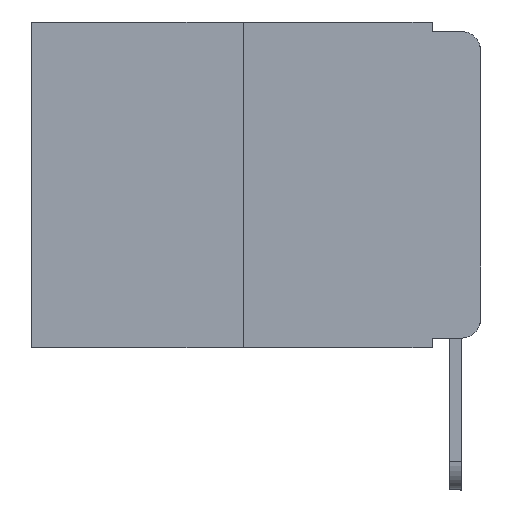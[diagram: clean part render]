
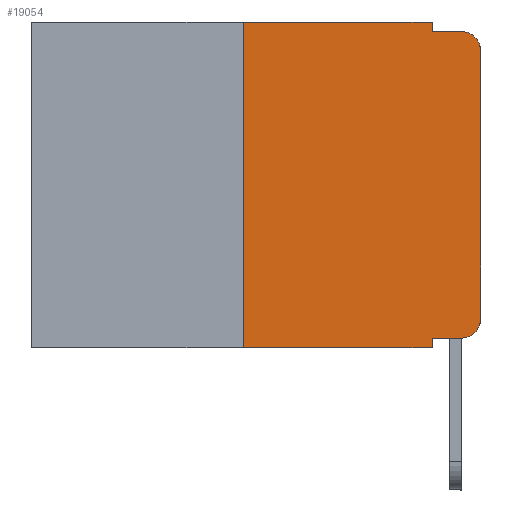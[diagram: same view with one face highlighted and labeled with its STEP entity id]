
A CAD part, left-side view. The second image highlights one B-rep face of the part: STEP entity #19054.
In plain terms, the highlighted planar face has unit normal (-1, 0, 0).
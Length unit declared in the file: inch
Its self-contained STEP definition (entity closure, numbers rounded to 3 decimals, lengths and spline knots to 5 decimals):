
#130 = VECTOR ( 'NONE', #16794, 39.37008 ) ;
#879 = LINE ( 'NONE', #5907, #19585 ) ;
#1122 = VECTOR ( 'NONE', #14082, 39.37008 ) ;
#1178 = VERTEX_POINT ( 'NONE', #13320 ) ;
#1684 = VECTOR ( 'NONE', #13153, 39.37008 ) ;
#2088 = CARTESIAN_POINT ( 'NONE',  ( 0., 0.051, -0.343 ) ) ;
#2218 = DIRECTION ( 'NONE',  ( 0., -1., 0. ) ) ;
#2637 = DIRECTION ( 'NONE',  ( 0., 0., -1. ) ) ;
#2649 = ORIENTED_EDGE ( 'NONE', *, *, #18471, .F. ) ;
#2933 = AXIS2_PLACEMENT_3D ( 'NONE', #17902, #2982, #14634 ) ;
#2982 = DIRECTION ( 'NONE',  ( -1., 0., 0. ) ) ;
#2997 = DIRECTION ( 'NONE',  ( 0., 0., -1. ) ) ;
#3019 = CARTESIAN_POINT ( 'NONE',  ( 0., 0.02, -0.333 ) ) ;
#3171 = VERTEX_POINT ( 'NONE', #12402 ) ;
#3204 = LINE ( 'NONE', #9836, #130 ) ;
#3533 = VECTOR ( 'NONE', #2997, 39.37008 ) ;
#4018 = EDGE_CURVE ( 'NONE', #15065, #11199, #5393, .T. ) ;
#4081 = CARTESIAN_POINT ( 'NONE',  ( 0., 0.051, -0.333 ) ) ;
#4201 = LINE ( 'NONE', #12363, #8523 ) ;
#4437 = VECTOR ( 'NONE', #2218, 39.37008 ) ;
#4520 = CARTESIAN_POINT ( 'NONE',  ( 0., 0.051, 0. ) ) ;
#4882 = VERTEX_POINT ( 'NONE', #17727 ) ;
#5393 = LINE ( 'NONE', #19218, #4437 ) ;
#5612 = DIRECTION ( 'NONE',  ( 0., 0., 1. ) ) ;
#5907 = CARTESIAN_POINT ( 'NONE',  ( 0., 0.051, 0. ) ) ;
#6014 = LINE ( 'NONE', #7534, #1122 ) ;
#6419 = DIRECTION ( 'NONE',  ( 1., 0., 0. ) ) ;
#6488 = CARTESIAN_POINT ( 'NONE',  ( 0., 0.051, -0.01 ) ) ;
#6549 = CARTESIAN_POINT ( 'NONE',  ( 0., 0.02, -0.03 ) ) ;
#6575 = CARTESIAN_POINT ( 'NONE',  ( 0., 0.051, 0. ) ) ;
#6661 = EDGE_CURVE ( 'NONE', #12435, #9947, #6906, .T. ) ;
#6898 = ORIENTED_EDGE ( 'NONE', *, *, #6661, .F. ) ;
#6906 = LINE ( 'NONE', #6488, #1684 ) ;
#7318 = CARTESIAN_POINT ( 'NONE',  ( 0., 0.02, -0.01 ) ) ;
#7534 = CARTESIAN_POINT ( 'NONE',  ( 0., 0.25, 0. ) ) ;
#7578 = CARTESIAN_POINT ( 'NONE',  ( 0., 0.25, -0.343 ) ) ;
#7665 = CARTESIAN_POINT ( 'NONE',  ( 0., 0.25, 0. ) ) ;
#7877 = VERTEX_POINT ( 'NONE', #3019 ) ;
#8114 = ORIENTED_EDGE ( 'NONE', *, *, #13920, .F. ) ;
#8523 = VECTOR ( 'NONE', #5612, 39.37008 ) ;
#9652 = VERTEX_POINT ( 'NONE', #7665 ) ;
#9836 = CARTESIAN_POINT ( 'NONE',  ( 0., 0.473, 0. ) ) ;
#9839 = ORIENTED_EDGE ( 'NONE', *, *, #15367, .T. ) ;
#9947 = VERTEX_POINT ( 'NONE', #7318 ) ;
#10528 = ORIENTED_EDGE ( 'NONE', *, *, #4018, .T. ) ;
#11019 = VECTOR ( 'NONE', #19105, 39.37008 ) ;
#11199 = VERTEX_POINT ( 'NONE', #2088 ) ;
#12363 = CARTESIAN_POINT ( 'NONE',  ( 0., 0., 0. ) ) ;
#12402 = CARTESIAN_POINT ( 'NONE',  ( 0., 0., -0.313 ) ) ;
#12435 = VERTEX_POINT ( 'NONE', #17462 ) ;
#12578 = LINE ( 'NONE', #4081, #11019 ) ;
#12999 = DIRECTION ( 'NONE',  ( 0., 0., -1. ) ) ;
#13153 = DIRECTION ( 'NONE',  ( 0., -1., 0. ) ) ;
#13306 = EDGE_LOOP ( 'NONE', ( #21253, #15072, #6898, #19586, #8114, #2649, #10528, #14712, #9839, #20119 ) ) ;
#13320 = CARTESIAN_POINT ( 'NONE',  ( 0., 0., -0.03 ) ) ;
#13336 = AXIS2_PLACEMENT_3D ( 'NONE', #6549, #14953, #12999 ) ;
#13729 = EDGE_CURVE ( 'NONE', #7877, #3171, #19641, .T. ) ;
#13920 = EDGE_CURVE ( 'NONE', #9652, #18074, #3204, .T. ) ;
#14082 = DIRECTION ( 'NONE',  ( 0., 0., 1. ) ) ;
#14634 = DIRECTION ( 'NONE',  ( 0., 0., -1. ) ) ;
#14712 = ORIENTED_EDGE ( 'NONE', *, *, #18508, .F. ) ;
#14953 = DIRECTION ( 'NONE',  ( -1., 0., 0. ) ) ;
#15065 = VERTEX_POINT ( 'NONE', #7578 ) ;
#15072 = ORIENTED_EDGE ( 'NONE', *, *, #18579, .T. ) ;
#15367 = EDGE_CURVE ( 'NONE', #4882, #7877, #12578, .T. ) ;
#16794 = DIRECTION ( 'NONE',  ( 0., -1., 0. ) ) ;
#16840 = EDGE_CURVE ( 'NONE', #18074, #12435, #18342, .T. ) ;
#17462 = CARTESIAN_POINT ( 'NONE',  ( 0., 0.051, -0.01 ) ) ;
#17727 = CARTESIAN_POINT ( 'NONE',  ( 0., 0.051, -0.333 ) ) ;
#17863 = DIRECTION ( 'NONE',  ( 0., 0., -1. ) ) ;
#17902 = CARTESIAN_POINT ( 'NONE',  ( 0., 0.02, -0.313 ) ) ;
#18074 = VERTEX_POINT ( 'NONE', #4520 ) ;
#18342 = LINE ( 'NONE', #6575, #3533 ) ;
#18471 = EDGE_CURVE ( 'NONE', #15065, #9652, #6014, .T. ) ;
#18508 = EDGE_CURVE ( 'NONE', #4882, #11199, #879, .T. ) ;
#18564 = AXIS2_PLACEMENT_3D ( 'NONE', #21360, #6419, #17863 ) ;
#18579 = EDGE_CURVE ( 'NONE', #1178, #9947, #21354, .T. ) ;
#19054 = ADVANCED_FACE ( 'NONE', ( #19933 ), #21469, .F. ) ;
#19105 = DIRECTION ( 'NONE',  ( 0., -1., 0. ) ) ;
#19218 = CARTESIAN_POINT ( 'NONE',  ( 0., 0.473, -0.343 ) ) ;
#19585 = VECTOR ( 'NONE', #2637, 39.37008 ) ;
#19586 = ORIENTED_EDGE ( 'NONE', *, *, #16840, .F. ) ;
#19641 = CIRCLE ( 'NONE', #2933, 0.02 ) ;
#19933 = FACE_OUTER_BOUND ( 'NONE', #13306, .T. ) ;
#20119 = ORIENTED_EDGE ( 'NONE', *, *, #13729, .T. ) ;
#20955 = EDGE_CURVE ( 'NONE', #3171, #1178, #4201, .T. ) ;
#21253 = ORIENTED_EDGE ( 'NONE', *, *, #20955, .T. ) ;
#21354 = CIRCLE ( 'NONE', #13336, 0.02 ) ;
#21360 = CARTESIAN_POINT ( 'NONE',  ( 0., 0.473, 0. ) ) ;
#21469 = PLANE ( 'NONE',  #18564 ) ;
